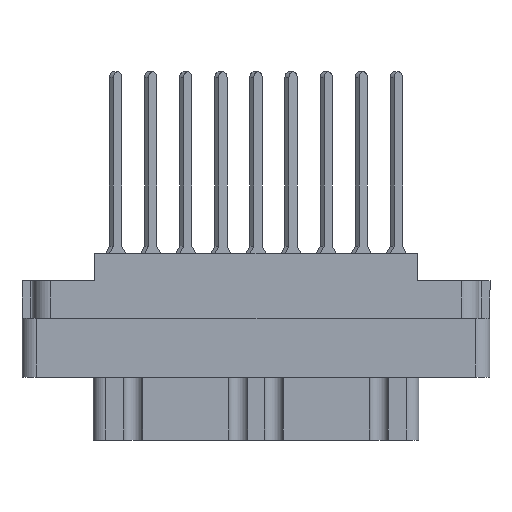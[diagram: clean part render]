
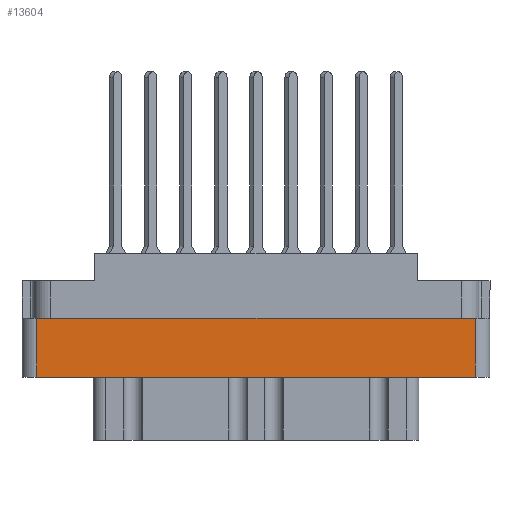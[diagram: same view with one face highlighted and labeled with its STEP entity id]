
A CAD part, front view. The second image highlights one B-rep face of the part: STEP entity #13604.
In plain terms, the highlighted planar face has unit normal (0, -1, 0).
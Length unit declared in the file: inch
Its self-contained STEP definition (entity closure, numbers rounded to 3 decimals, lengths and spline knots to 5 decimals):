
#509 = LINE ( 'NONE', #23356, #5542 ) ;
#2164 = PLANE ( 'NONE',  #29084 ) ;
#3257 = CARTESIAN_POINT ( 'NONE',  ( -1., -0.438, -0.277 ) ) ;
#4035 = CARTESIAN_POINT ( 'NONE',  ( -0.938, -0.438, -0.798 ) ) ;
#4202 = ORIENTED_EDGE ( 'NONE', *, *, #6121, .F. ) ;
#4682 = DIRECTION ( 'NONE',  ( 0., 0., 1. ) ) ;
#5542 = VECTOR ( 'NONE', #13069, 39.37008 ) ;
#6121 = EDGE_CURVE ( 'NONE', #24847, #14616, #11877, .T. ) ;
#6494 = LINE ( 'NONE', #3257, #28752 ) ;
#7756 = EDGE_CURVE ( 'NONE', #14616, #17018, #6494, .T. ) ;
#9164 = DIRECTION ( 'NONE',  ( 0., -1., 0. ) ) ;
#11877 = LINE ( 'NONE', #4035, #31555 ) ;
#11952 = CARTESIAN_POINT ( 'NONE',  ( -0.938, -0.438, -0.798 ) ) ;
#12376 = CARTESIAN_POINT ( 'NONE',  ( 0.938, -0.438, -0.798 ) ) ;
#13069 = DIRECTION ( 'NONE',  ( -1., 0., 0. ) ) ;
#13604 = ADVANCED_FACE ( 'NONE', ( #22238 ), #2164, .T. ) ;
#14393 = DIRECTION ( 'NONE',  ( 0., 0., -1. ) ) ;
#14616 = VERTEX_POINT ( 'NONE', #22320 ) ;
#15048 = ORIENTED_EDGE ( 'NONE', *, *, #7756, .F. ) ;
#16035 = CARTESIAN_POINT ( 'NONE',  ( 0.938, -0.438, -0.529 ) ) ;
#16100 = CARTESIAN_POINT ( 'NONE',  ( 0.938, -0.438, -0.277 ) ) ;
#16928 = DIRECTION ( 'NONE',  ( 0., 0., 1. ) ) ;
#16930 = CARTESIAN_POINT ( 'NONE',  ( -0.938, -0.438, -0.529 ) ) ;
#17018 = VERTEX_POINT ( 'NONE', #16100 ) ;
#17107 = ORIENTED_EDGE ( 'NONE', *, *, #28637, .T. ) ;
#17547 = VECTOR ( 'NONE', #16928, 39.37008 ) ;
#19723 = LINE ( 'NONE', #12376, #17547 ) ;
#21691 = EDGE_LOOP ( 'NONE', ( #4202, #29470, #17107, #15048 ) ) ;
#22100 = VERTEX_POINT ( 'NONE', #16035 ) ;
#22238 = FACE_OUTER_BOUND ( 'NONE', #21691, .T. ) ;
#22320 = CARTESIAN_POINT ( 'NONE',  ( -0.938, -0.438, -0.277 ) ) ;
#23356 = CARTESIAN_POINT ( 'NONE',  ( 0.938, -0.438, -0.529 ) ) ;
#24089 = EDGE_CURVE ( 'NONE', #22100, #24847, #509, .T. ) ;
#24847 = VERTEX_POINT ( 'NONE', #16930 ) ;
#25615 = DIRECTION ( 'NONE',  ( 1., 0., 0. ) ) ;
#28637 = EDGE_CURVE ( 'NONE', #22100, #17018, #19723, .T. ) ;
#28752 = VECTOR ( 'NONE', #25615, 39.37008 ) ;
#29084 = AXIS2_PLACEMENT_3D ( 'NONE', #11952, #9164, #14393 ) ;
#29470 = ORIENTED_EDGE ( 'NONE', *, *, #24089, .F. ) ;
#31555 = VECTOR ( 'NONE', #4682, 39.37008 ) ;
